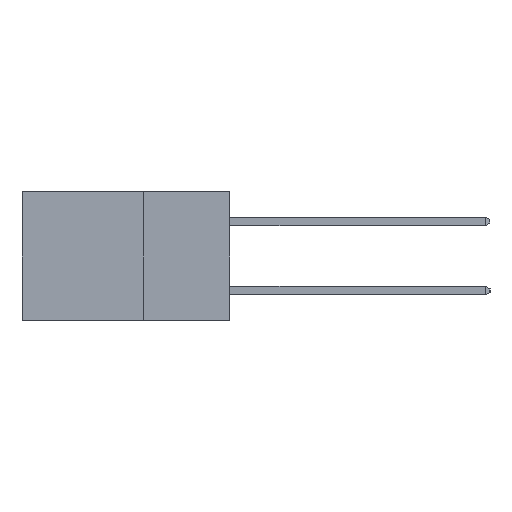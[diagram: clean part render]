
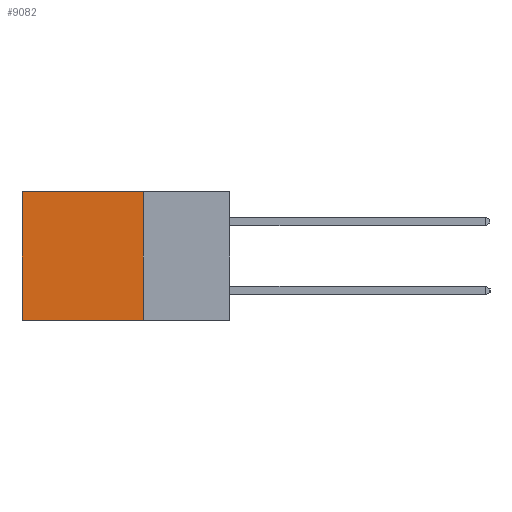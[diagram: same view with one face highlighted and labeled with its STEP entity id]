
A CAD part, left-side view. The second image highlights one B-rep face of the part: STEP entity #9082.
In plain terms, the highlighted planar face has unit normal (-1, 0, 0).
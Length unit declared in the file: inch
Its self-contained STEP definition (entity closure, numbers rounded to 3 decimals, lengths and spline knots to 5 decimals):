
#313 = DIRECTION ( 'NONE',  ( 1., 0., 0. ) ) ;
#440 = VECTOR ( 'NONE', #8896, 39.37008 ) ;
#1093 = VERTEX_POINT ( 'NONE', #9076 ) ;
#1254 = AXIS2_PLACEMENT_3D ( 'NONE', #3186, #313, #7107 ) ;
#1413 = EDGE_CURVE ( 'NONE', #1093, #6909, #10390, .T. ) ;
#1575 = ORIENTED_EDGE ( 'NONE', *, *, #5228, .T. ) ;
#1641 = EDGE_CURVE ( 'NONE', #9561, #3177, #3008, .T. ) ;
#1808 = DIRECTION ( 'NONE',  ( 0., 0., -1. ) ) ;
#2142 = CARTESIAN_POINT ( 'NONE',  ( 0.2615, 0.25, -0.37 ) ) ;
#2304 = EDGE_CURVE ( 'NONE', #6909, #3177, #2542, .T. ) ;
#2542 = LINE ( 'NONE', #9378, #4810 ) ;
#2545 = ORIENTED_EDGE ( 'NONE', *, *, #2304, .F. ) ;
#3008 = LINE ( 'NONE', #8087, #440 ) ;
#3177 = VERTEX_POINT ( 'NONE', #7103 ) ;
#3186 = CARTESIAN_POINT ( 'NONE',  ( 0.2615, 0.25, -0.37 ) ) ;
#3288 = VECTOR ( 'NONE', #11665, 39.37008 ) ;
#4810 = VECTOR ( 'NONE', #9354, 39.37008 ) ;
#5228 = EDGE_CURVE ( 'NONE', #1093, #9561, #5912, .T. ) ;
#5307 = CARTESIAN_POINT ( 'NONE',  ( 0.2615, 0.25, 0. ) ) ;
#5467 = EDGE_LOOP ( 'NONE', ( #9313, #2545, #10013, #1575 ) ) ;
#5912 = LINE ( 'NONE', #5307, #3288 ) ;
#5965 = FACE_OUTER_BOUND ( 'NONE', #5467, .T. ) ;
#6909 = VERTEX_POINT ( 'NONE', #10301 ) ;
#7103 = CARTESIAN_POINT ( 'NONE',  ( 0.2615, 0.6, -0.37 ) ) ;
#7107 = DIRECTION ( 'NONE',  ( 0., 0., -1. ) ) ;
#7694 = CARTESIAN_POINT ( 'NONE',  ( 0.2615, 0.6, 0. ) ) ;
#8087 = CARTESIAN_POINT ( 'NONE',  ( 0.2615, 0.6, -0.37 ) ) ;
#8896 = DIRECTION ( 'NONE',  ( 0., 0., -1. ) ) ;
#9076 = CARTESIAN_POINT ( 'NONE',  ( 0.2615, 0.25, 0. ) ) ;
#9082 = ADVANCED_FACE ( 'NONE', ( #5965 ), #10705, .F. ) ;
#9313 = ORIENTED_EDGE ( 'NONE', *, *, #1641, .T. ) ;
#9354 = DIRECTION ( 'NONE',  ( 0., 1., 0. ) ) ;
#9378 = CARTESIAN_POINT ( 'NONE',  ( 0.2615, 0.25, -0.37 ) ) ;
#9561 = VERTEX_POINT ( 'NONE', #7694 ) ;
#10013 = ORIENTED_EDGE ( 'NONE', *, *, #1413, .F. ) ;
#10118 = VECTOR ( 'NONE', #1808, 39.37008 ) ;
#10301 = CARTESIAN_POINT ( 'NONE',  ( 0.2615, 0.25, -0.37 ) ) ;
#10390 = LINE ( 'NONE', #2142, #10118 ) ;
#10705 = PLANE ( 'NONE',  #1254 ) ;
#11665 = DIRECTION ( 'NONE',  ( 0., 1., 0. ) ) ;
